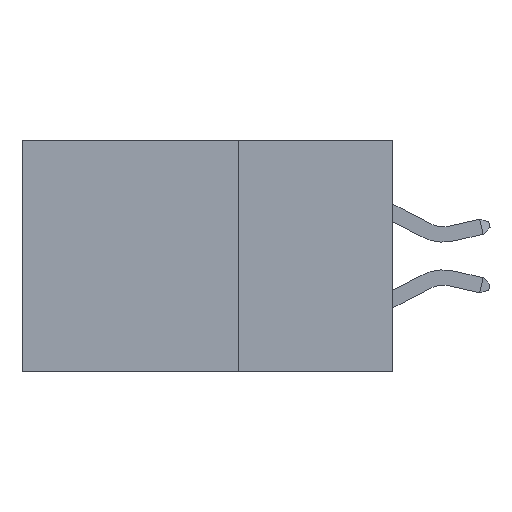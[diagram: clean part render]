
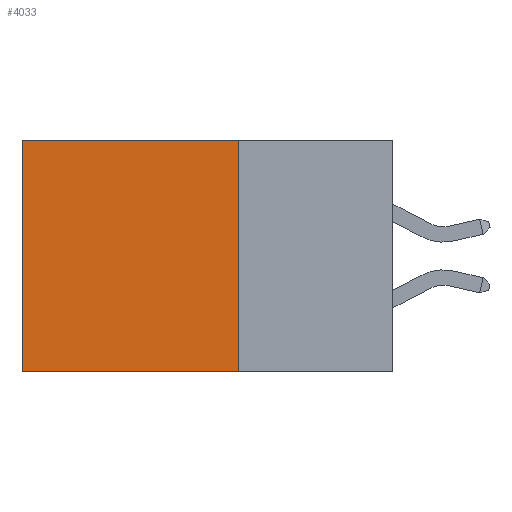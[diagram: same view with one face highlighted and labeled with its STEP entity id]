
A CAD part, left-side view. The second image highlights one B-rep face of the part: STEP entity #4033.
In plain terms, the highlighted planar face has unit normal (-1, 0, 0).
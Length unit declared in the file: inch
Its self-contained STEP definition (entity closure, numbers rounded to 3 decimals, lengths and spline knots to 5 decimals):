
#90 = LINE ( 'NONE', #895, #5644 ) ;
#208 = ORIENTED_EDGE ( 'NONE', *, *, #9086, .T. ) ;
#235 = CARTESIAN_POINT ( 'NONE',  ( 0.2875, 0.25, -0.375 ) ) ;
#309 = VERTEX_POINT ( 'NONE', #10171 ) ;
#311 = CARTESIAN_POINT ( 'NONE',  ( 0.2875, 0.6, 0. ) ) ;
#458 = DIRECTION ( 'NONE',  ( 0., 0., -1. ) ) ;
#895 = CARTESIAN_POINT ( 'NONE',  ( 0.2875, 0.25, -0.375 ) ) ;
#1263 = DIRECTION ( 'NONE',  ( 0., 1., 0. ) ) ;
#1546 = VERTEX_POINT ( 'NONE', #1947 ) ;
#1947 = CARTESIAN_POINT ( 'NONE',  ( 0.2875, 0.25, 0. ) ) ;
#2756 = LINE ( 'NONE', #235, #9919 ) ;
#2957 = CARTESIAN_POINT ( 'NONE',  ( 0.2875, 0.25, -0.375 ) ) ;
#3536 = VECTOR ( 'NONE', #1263, 39.37008 ) ;
#4033 = ADVANCED_FACE ( 'NONE', ( #6475 ), #12340, .F. ) ;
#5128 = ORIENTED_EDGE ( 'NONE', *, *, #10330, .T. ) ;
#5644 = VECTOR ( 'NONE', #13009, 39.37008 ) ;
#5924 = ORIENTED_EDGE ( 'NONE', *, *, #11470, .F. ) ;
#6000 = VECTOR ( 'NONE', #11195, 39.37008 ) ;
#6475 = FACE_OUTER_BOUND ( 'NONE', #12571, .T. ) ;
#7846 = CARTESIAN_POINT ( 'NONE',  ( 0.2875, 0.6, -0.375 ) ) ;
#8143 = CARTESIAN_POINT ( 'NONE',  ( 0.2875, 0.25, 0. ) ) ;
#8189 = AXIS2_PLACEMENT_3D ( 'NONE', #2957, #11117, #14208 ) ;
#9086 = EDGE_CURVE ( 'NONE', #1546, #10073, #14933, .T. ) ;
#9919 = VECTOR ( 'NONE', #458, 39.37008 ) ;
#10073 = VERTEX_POINT ( 'NONE', #311 ) ;
#10121 = LINE ( 'NONE', #7846, #6000 ) ;
#10171 = CARTESIAN_POINT ( 'NONE',  ( 0.2875, 0.6, -0.375 ) ) ;
#10330 = EDGE_CURVE ( 'NONE', #10073, #309, #10121, .T. ) ;
#11117 = DIRECTION ( 'NONE',  ( 1., 0., 0. ) ) ;
#11195 = DIRECTION ( 'NONE',  ( 0., 0., -1. ) ) ;
#11470 = EDGE_CURVE ( 'NONE', #1546, #13246, #2756, .T. ) ;
#12163 = EDGE_CURVE ( 'NONE', #13246, #309, #90, .T. ) ;
#12340 = PLANE ( 'NONE',  #8189 ) ;
#12515 = CARTESIAN_POINT ( 'NONE',  ( 0.2875, 0.25, -0.375 ) ) ;
#12571 = EDGE_LOOP ( 'NONE', ( #5128, #13590, #5924, #208 ) ) ;
#13009 = DIRECTION ( 'NONE',  ( 0., 1., 0. ) ) ;
#13246 = VERTEX_POINT ( 'NONE', #12515 ) ;
#13590 = ORIENTED_EDGE ( 'NONE', *, *, #12163, .F. ) ;
#14208 = DIRECTION ( 'NONE',  ( 0., 0., -1. ) ) ;
#14933 = LINE ( 'NONE', #8143, #3536 ) ;
